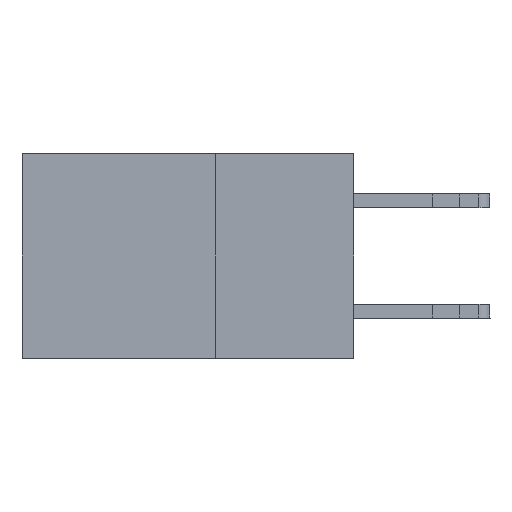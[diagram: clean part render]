
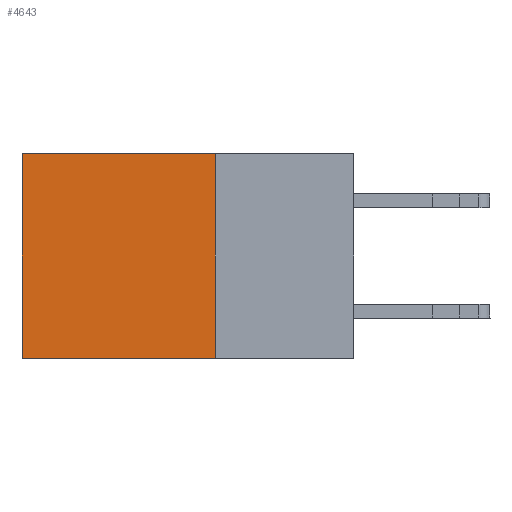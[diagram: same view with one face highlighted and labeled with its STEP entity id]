
A CAD part, left-side view. The second image highlights one B-rep face of the part: STEP entity #4643.
In plain terms, the highlighted planar face has unit normal (-1, 0, 0).
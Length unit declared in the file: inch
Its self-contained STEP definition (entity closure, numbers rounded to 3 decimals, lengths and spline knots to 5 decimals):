
#4 = EDGE_LOOP ( 'NONE', ( #18847, #5101, #22967, #13719 ) ) ;
#782 = EDGE_CURVE ( 'NONE', #4224, #11529, #1065, .T. ) ;
#1001 = CARTESIAN_POINT ( 'NONE',  ( 0.2875, 0.25, 0. ) ) ;
#1065 = LINE ( 'NONE', #13985, #14889 ) ;
#1832 = CARTESIAN_POINT ( 'NONE',  ( 0.2875, 0.6, -0.37 ) ) ;
#3885 = LINE ( 'NONE', #1001, #22770 ) ;
#4224 = VERTEX_POINT ( 'NONE', #13468 ) ;
#4342 = CARTESIAN_POINT ( 'NONE',  ( 0.2875, 0.6, 0. ) ) ;
#4597 = CARTESIAN_POINT ( 'NONE',  ( 0.2875, 0.6, 0. ) ) ;
#4643 = ADVANCED_FACE ( 'NONE', ( #17634 ), #10625, .F. ) ;
#4786 = VERTEX_POINT ( 'NONE', #9167 ) ;
#5101 = ORIENTED_EDGE ( 'NONE', *, *, #782, .F. ) ;
#6161 = CARTESIAN_POINT ( 'NONE',  ( 0.2875, 0.25, 0. ) ) ;
#6203 = DIRECTION ( 'NONE',  ( 0., 0., -1. ) ) ;
#7116 = DIRECTION ( 'NONE',  ( 0., 1., 0. ) ) ;
#9167 = CARTESIAN_POINT ( 'NONE',  ( 0.2875, 0.25, 0. ) ) ;
#10058 = DIRECTION ( 'NONE',  ( 0., 1., 0. ) ) ;
#10560 = EDGE_CURVE ( 'NONE', #4786, #19952, #18219, .T. ) ;
#10573 = EDGE_CURVE ( 'NONE', #4786, #4224, #3885, .T. ) ;
#10625 = PLANE ( 'NONE',  #12373 ) ;
#11529 = VERTEX_POINT ( 'NONE', #1832 ) ;
#11806 = EDGE_CURVE ( 'NONE', #19952, #11529, #12647, .T. ) ;
#12373 = AXIS2_PLACEMENT_3D ( 'NONE', #21118, #22826, #12412 ) ;
#12412 = DIRECTION ( 'NONE',  ( 0., 0., -1. ) ) ;
#12647 = LINE ( 'NONE', #4342, #20836 ) ;
#13468 = CARTESIAN_POINT ( 'NONE',  ( 0.2875, 0.25, -0.37 ) ) ;
#13505 = VECTOR ( 'NONE', #10058, 39.37008 ) ;
#13719 = ORIENTED_EDGE ( 'NONE', *, *, #10560, .T. ) ;
#13985 = CARTESIAN_POINT ( 'NONE',  ( 0.2875, 0.25, -0.37 ) ) ;
#14889 = VECTOR ( 'NONE', #7116, 39.37008 ) ;
#17220 = DIRECTION ( 'NONE',  ( 0., 0., -1. ) ) ;
#17634 = FACE_OUTER_BOUND ( 'NONE', #4, .T. ) ;
#18219 = LINE ( 'NONE', #6161, #13505 ) ;
#18847 = ORIENTED_EDGE ( 'NONE', *, *, #11806, .T. ) ;
#19952 = VERTEX_POINT ( 'NONE', #4597 ) ;
#20836 = VECTOR ( 'NONE', #6203, 39.37008 ) ;
#21118 = CARTESIAN_POINT ( 'NONE',  ( 0.2875, 0.25, 0. ) ) ;
#22770 = VECTOR ( 'NONE', #17220, 39.37008 ) ;
#22826 = DIRECTION ( 'NONE',  ( 1., 0., 0. ) ) ;
#22967 = ORIENTED_EDGE ( 'NONE', *, *, #10573, .F. ) ;
